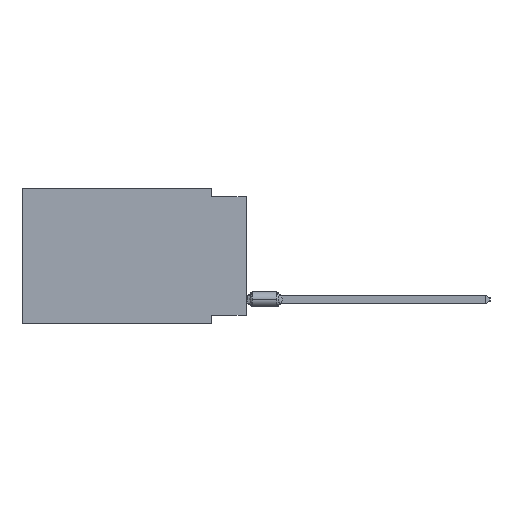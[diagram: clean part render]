
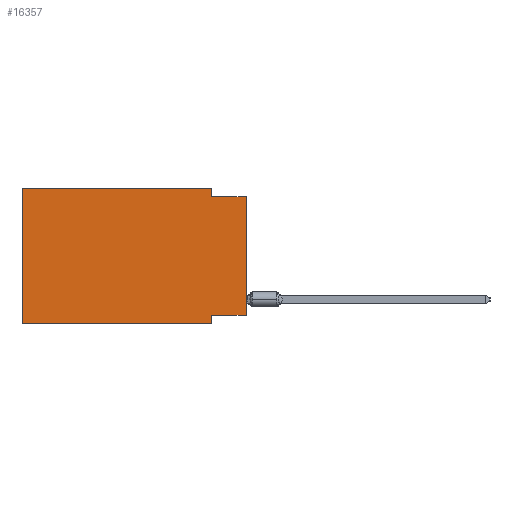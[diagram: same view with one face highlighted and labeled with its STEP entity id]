
A CAD part, left-side view. The second image highlights one B-rep face of the part: STEP entity #16357.
In plain terms, the highlighted planar face has unit normal (-1, 0, 0).
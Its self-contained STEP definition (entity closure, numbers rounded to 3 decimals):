
#307 = VECTOR ( 'NONE', #23866, 1000. ) ;
#869 = ORIENTED_EDGE ( 'NONE', *, *, #46256, .F. ) ;
#2108 = LINE ( 'NONE', #29691, #56252 ) ;
#2966 = VERTEX_POINT ( 'NONE', #47954 ) ;
#3178 = CARTESIAN_POINT ( 'NONE',  ( 0., 2.54, -9.906 ) ) ;
#4204 = DIRECTION ( 'NONE',  ( 0., -1., 0. ) ) ;
#5587 = LINE ( 'NONE', #18460, #307 ) ;
#6144 = DIRECTION ( 'NONE',  ( 0., 0., 1. ) ) ;
#6499 = DIRECTION ( 'NONE',  ( 0., 0., -1. ) ) ;
#6508 = DIRECTION ( 'NONE',  ( 0., 0., -1. ) ) ;
#10191 = DIRECTION ( 'NONE',  ( 0., 0., 1. ) ) ;
#10855 = CARTESIAN_POINT ( 'NONE',  ( 0., 16.383, 0. ) ) ;
#10894 = EDGE_CURVE ( 'NONE', #22639, #2966, #2108, .T. ) ;
#11107 = CARTESIAN_POINT ( 'NONE',  ( 0., 0., -9.271 ) ) ;
#12048 = FACE_OUTER_BOUND ( 'NONE', #25175, .T. ) ;
#12126 = ORIENTED_EDGE ( 'NONE', *, *, #13236, .F. ) ;
#12144 = ORIENTED_EDGE ( 'NONE', *, *, #58943, .F. ) ;
#12877 = AXIS2_PLACEMENT_3D ( 'NONE', #10855, #38759, #34853 ) ;
#13236 = EDGE_CURVE ( 'NONE', #51355, #16919, #5587, .T. ) ;
#14640 = CARTESIAN_POINT ( 'NONE',  ( 0., 2.54, -0.635 ) ) ;
#15135 = CARTESIAN_POINT ( 'NONE',  ( 0., 0., 0. ) ) ;
#16357 = ADVANCED_FACE ( 'NONE', ( #12048 ), #16538, .F. ) ;
#16538 = PLANE ( 'NONE',  #12877 ) ;
#16919 = VERTEX_POINT ( 'NONE', #35896 ) ;
#17247 = ORIENTED_EDGE ( 'NONE', *, *, #10894, .T. ) ;
#18460 = CARTESIAN_POINT ( 'NONE',  ( 0., 0., -0.635 ) ) ;
#19486 = LINE ( 'NONE', #47981, #46534 ) ;
#20980 = CARTESIAN_POINT ( 'NONE',  ( 0., 16.383, -9.906 ) ) ;
#21755 = VECTOR ( 'NONE', #4204, 1000. ) ;
#22639 = VERTEX_POINT ( 'NONE', #20980 ) ;
#23866 = DIRECTION ( 'NONE',  ( 0., -1., 0. ) ) ;
#24095 = VECTOR ( 'NONE', #6508, 1000. ) ;
#24310 = LINE ( 'NONE', #11107, #27809 ) ;
#24390 = VERTEX_POINT ( 'NONE', #57551 ) ;
#24663 = CARTESIAN_POINT ( 'NONE',  ( 0., 2.54, -9.271 ) ) ;
#25080 = LINE ( 'NONE', #3178, #24095 ) ;
#25175 = EDGE_LOOP ( 'NONE', ( #32077, #12126, #25919, #869, #12144, #17247, #32994, #42861 ) ) ;
#25919 = ORIENTED_EDGE ( 'NONE', *, *, #35311, .F. ) ;
#27809 = VECTOR ( 'NONE', #56143, 1000. ) ;
#27927 = EDGE_CURVE ( 'NONE', #31430, #16919, #47245, .T. ) ;
#29691 = CARTESIAN_POINT ( 'NONE',  ( 0., 16.383, -9.906 ) ) ;
#30414 = VECTOR ( 'NONE', #6144, 1000. ) ;
#31430 = VERTEX_POINT ( 'NONE', #39645 ) ;
#32077 = ORIENTED_EDGE ( 'NONE', *, *, #27927, .T. ) ;
#32994 = ORIENTED_EDGE ( 'NONE', *, *, #33718, .F. ) ;
#33718 = EDGE_CURVE ( 'NONE', #49126, #2966, #25080, .T. ) ;
#33784 = CARTESIAN_POINT ( 'NONE',  ( 0., 2.54, 0. ) ) ;
#34853 = DIRECTION ( 'NONE',  ( 0., 0., -1. ) ) ;
#35311 = EDGE_CURVE ( 'NONE', #24390, #51355, #56601, .T. ) ;
#35896 = CARTESIAN_POINT ( 'NONE',  ( 0., 0., -0.635 ) ) ;
#36023 = CARTESIAN_POINT ( 'NONE',  ( 0., 16.383, 0. ) ) ;
#38759 = DIRECTION ( 'NONE',  ( 1., 0., 0. ) ) ;
#39645 = CARTESIAN_POINT ( 'NONE',  ( 0., 0., -9.271 ) ) ;
#39766 = CARTESIAN_POINT ( 'NONE',  ( 0., 16.383, 0. ) ) ;
#41357 = VECTOR ( 'NONE', #6499, 1000. ) ;
#42861 = ORIENTED_EDGE ( 'NONE', *, *, #50875, .F. ) ;
#45308 = LINE ( 'NONE', #36023, #21755 ) ;
#46256 = EDGE_CURVE ( 'NONE', #53960, #24390, #45308, .T. ) ;
#46534 = VECTOR ( 'NONE', #10191, 1000. ) ;
#47245 = LINE ( 'NONE', #15135, #30414 ) ;
#47954 = CARTESIAN_POINT ( 'NONE',  ( 0., 2.54, -9.906 ) ) ;
#47981 = CARTESIAN_POINT ( 'NONE',  ( 0., 16.383, 0. ) ) ;
#48310 = DIRECTION ( 'NONE',  ( 0., -1., 0. ) ) ;
#49126 = VERTEX_POINT ( 'NONE', #24663 ) ;
#50875 = EDGE_CURVE ( 'NONE', #31430, #49126, #24310, .T. ) ;
#51355 = VERTEX_POINT ( 'NONE', #14640 ) ;
#53960 = VERTEX_POINT ( 'NONE', #39766 ) ;
#56143 = DIRECTION ( 'NONE',  ( 0., 1., 0. ) ) ;
#56252 = VECTOR ( 'NONE', #48310, 1000. ) ;
#56601 = LINE ( 'NONE', #33784, #41357 ) ;
#57551 = CARTESIAN_POINT ( 'NONE',  ( 0., 2.54, 0. ) ) ;
#58943 = EDGE_CURVE ( 'NONE', #22639, #53960, #19486, .T. ) ;
